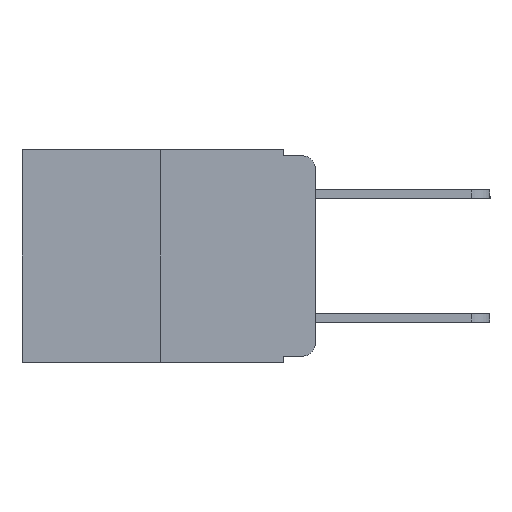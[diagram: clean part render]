
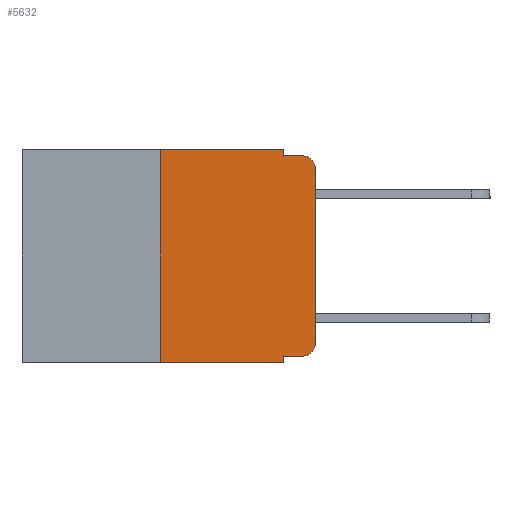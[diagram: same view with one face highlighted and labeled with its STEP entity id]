
A CAD part, left-side view. The second image highlights one B-rep face of the part: STEP entity #5632.
In plain terms, the highlighted planar face has unit normal (-1, 0, 0).
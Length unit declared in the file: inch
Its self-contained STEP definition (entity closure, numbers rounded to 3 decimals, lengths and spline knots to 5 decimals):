
#23 = DIRECTION ( 'NONE',  ( 0., 0., -1. ) ) ;
#94 = EDGE_CURVE ( 'NONE', #9691, #3349, #7929, .T. ) ;
#184 = VECTOR ( 'NONE', #1637, 39.37008 ) ;
#443 = DIRECTION ( 'NONE',  ( 0., -1., 0. ) ) ;
#707 = CARTESIAN_POINT ( 'NONE',  ( 0., 0., 0. ) ) ;
#891 = EDGE_CURVE ( 'NONE', #11151, #11703, #5564, .T. ) ;
#1611 = DIRECTION ( 'NONE',  ( 1., 0., 0. ) ) ;
#1637 = DIRECTION ( 'NONE',  ( 0., 0., -1. ) ) ;
#1639 = EDGE_CURVE ( 'NONE', #11703, #4674, #11117, .T. ) ;
#1683 = VERTEX_POINT ( 'NONE', #2670 ) ;
#1728 = CIRCLE ( 'NONE', #4755, 0.02 ) ;
#1909 = LINE ( 'NONE', #10342, #6723 ) ;
#1938 = VECTOR ( 'NONE', #9876, 39.37008 ) ;
#2224 = VECTOR ( 'NONE', #6646, 39.37008 ) ;
#2319 = CARTESIAN_POINT ( 'NONE',  ( 0., 0.051, 0. ) ) ;
#2609 = VECTOR ( 'NONE', #5099, 39.37008 ) ;
#2670 = CARTESIAN_POINT ( 'NONE',  ( 0., 0.02, -0.333 ) ) ;
#2672 = DIRECTION ( 'NONE',  ( -1., 0., 0. ) ) ;
#2720 = ORIENTED_EDGE ( 'NONE', *, *, #891, .F. ) ;
#2728 = CARTESIAN_POINT ( 'NONE',  ( 0., 0.051, -0.01 ) ) ;
#3116 = CARTESIAN_POINT ( 'NONE',  ( 0., 0.051, -0.343 ) ) ;
#3349 = VERTEX_POINT ( 'NONE', #9632 ) ;
#3373 = EDGE_CURVE ( 'NONE', #3349, #11151, #1909, .T. ) ;
#3384 = VECTOR ( 'NONE', #3503, 39.37008 ) ;
#3454 = CIRCLE ( 'NONE', #4156, 0.02 ) ;
#3503 = DIRECTION ( 'NONE',  ( 0., -1., 0. ) ) ;
#3581 = VECTOR ( 'NONE', #443, 39.37008 ) ;
#3601 = PLANE ( 'NONE',  #8474 ) ;
#3672 = EDGE_CURVE ( 'NONE', #6180, #4674, #1728, .T. ) ;
#3700 = DIRECTION ( 'NONE',  ( 0., 0., -1. ) ) ;
#3713 = VECTOR ( 'NONE', #3700, 39.37008 ) ;
#3864 = CARTESIAN_POINT ( 'NONE',  ( 0., 0., -0.03 ) ) ;
#3934 = VERTEX_POINT ( 'NONE', #11192 ) ;
#4034 = CARTESIAN_POINT ( 'NONE',  ( 0., 0.02, -0.01 ) ) ;
#4156 = AXIS2_PLACEMENT_3D ( 'NONE', #8346, #2672, #9201 ) ;
#4366 = EDGE_CURVE ( 'NONE', #3934, #6180, #11601, .T. ) ;
#4623 = CARTESIAN_POINT ( 'NONE',  ( 0., 0.473, 0. ) ) ;
#4673 = CARTESIAN_POINT ( 'NONE',  ( 0., 0.051, 0. ) ) ;
#4674 = VERTEX_POINT ( 'NONE', #4034 ) ;
#4755 = AXIS2_PLACEMENT_3D ( 'NONE', #6405, #6330, #23 ) ;
#4791 = CARTESIAN_POINT ( 'NONE',  ( 0., 0.051, -0.333 ) ) ;
#5099 = DIRECTION ( 'NONE',  ( 0., 0., 1. ) ) ;
#5213 = VERTEX_POINT ( 'NONE', #4791 ) ;
#5564 = LINE ( 'NONE', #2319, #184 ) ;
#5619 = FACE_OUTER_BOUND ( 'NONE', #7818, .T. ) ;
#5632 = ADVANCED_FACE ( 'NONE', ( #5619 ), #3601, .F. ) ;
#5865 = ORIENTED_EDGE ( 'NONE', *, *, #94, .F. ) ;
#6164 = LINE ( 'NONE', #6290, #3384 ) ;
#6180 = VERTEX_POINT ( 'NONE', #3864 ) ;
#6290 = CARTESIAN_POINT ( 'NONE',  ( 0., 0.473, -0.343 ) ) ;
#6330 = DIRECTION ( 'NONE',  ( -1., 0., 0. ) ) ;
#6385 = CARTESIAN_POINT ( 'NONE',  ( 0., 0.051, -0.333 ) ) ;
#6405 = CARTESIAN_POINT ( 'NONE',  ( 0., 0.02, -0.03 ) ) ;
#6646 = DIRECTION ( 'NONE',  ( 0., 0., 1. ) ) ;
#6723 = VECTOR ( 'NONE', #11154, 39.37008 ) ;
#7198 = EDGE_CURVE ( 'NONE', #9691, #7641, #6164, .T. ) ;
#7625 = ORIENTED_EDGE ( 'NONE', *, *, #11690, .F. ) ;
#7641 = VERTEX_POINT ( 'NONE', #3116 ) ;
#7818 = EDGE_LOOP ( 'NONE', ( #11399, #11262, #9802, #2720, #10336, #5865, #7913, #7625, #9050, #9569 ) ) ;
#7913 = ORIENTED_EDGE ( 'NONE', *, *, #7198, .T. ) ;
#7929 = LINE ( 'NONE', #10630, #2609 ) ;
#8087 = LINE ( 'NONE', #4673, #3713 ) ;
#8230 = CARTESIAN_POINT ( 'NONE',  ( 0., 0.25, -0.343 ) ) ;
#8303 = DIRECTION ( 'NONE',  ( 0., 0., -1. ) ) ;
#8346 = CARTESIAN_POINT ( 'NONE',  ( 0., 0.02, -0.313 ) ) ;
#8474 = AXIS2_PLACEMENT_3D ( 'NONE', #4623, #1611, #8303 ) ;
#9050 = ORIENTED_EDGE ( 'NONE', *, *, #11135, .T. ) ;
#9201 = DIRECTION ( 'NONE',  ( 0., 0., -1. ) ) ;
#9569 = ORIENTED_EDGE ( 'NONE', *, *, #10555, .T. ) ;
#9632 = CARTESIAN_POINT ( 'NONE',  ( 0., 0.25, 0. ) ) ;
#9691 = VERTEX_POINT ( 'NONE', #8230 ) ;
#9802 = ORIENTED_EDGE ( 'NONE', *, *, #1639, .F. ) ;
#9876 = DIRECTION ( 'NONE',  ( 0., -1., 0. ) ) ;
#9990 = CARTESIAN_POINT ( 'NONE',  ( 0., 0.051, 0. ) ) ;
#10336 = ORIENTED_EDGE ( 'NONE', *, *, #3373, .F. ) ;
#10342 = CARTESIAN_POINT ( 'NONE',  ( 0., 0.473, 0. ) ) ;
#10555 = EDGE_CURVE ( 'NONE', #1683, #3934, #3454, .T. ) ;
#10630 = CARTESIAN_POINT ( 'NONE',  ( 0., 0.25, 0. ) ) ;
#11045 = LINE ( 'NONE', #6385, #3581 ) ;
#11117 = LINE ( 'NONE', #11766, #1938 ) ;
#11135 = EDGE_CURVE ( 'NONE', #5213, #1683, #11045, .T. ) ;
#11151 = VERTEX_POINT ( 'NONE', #9990 ) ;
#11154 = DIRECTION ( 'NONE',  ( 0., -1., 0. ) ) ;
#11192 = CARTESIAN_POINT ( 'NONE',  ( 0., 0., -0.313 ) ) ;
#11262 = ORIENTED_EDGE ( 'NONE', *, *, #3672, .T. ) ;
#11399 = ORIENTED_EDGE ( 'NONE', *, *, #4366, .T. ) ;
#11601 = LINE ( 'NONE', #707, #2224 ) ;
#11690 = EDGE_CURVE ( 'NONE', #5213, #7641, #8087, .T. ) ;
#11703 = VERTEX_POINT ( 'NONE', #2728 ) ;
#11766 = CARTESIAN_POINT ( 'NONE',  ( 0., 0.051, -0.01 ) ) ;
